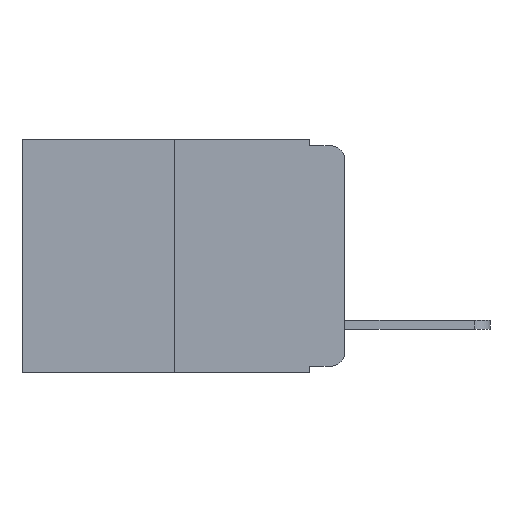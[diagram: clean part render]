
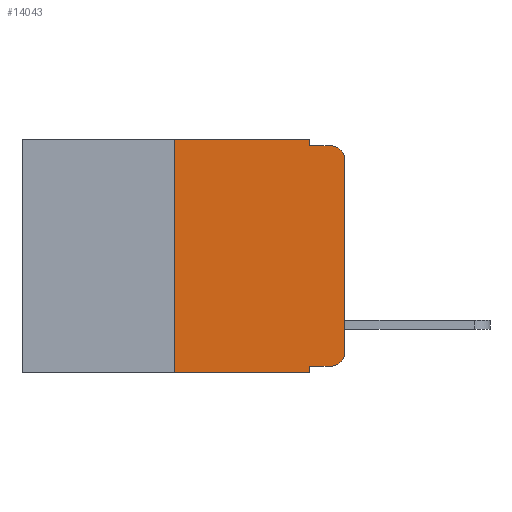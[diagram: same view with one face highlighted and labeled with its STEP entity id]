
A CAD part, left-side view. The second image highlights one B-rep face of the part: STEP entity #14043.
In plain terms, the highlighted planar face has unit normal (-1, 0, 0).
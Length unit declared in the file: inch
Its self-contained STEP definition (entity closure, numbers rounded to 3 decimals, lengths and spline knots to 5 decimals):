
#195 = EDGE_LOOP ( 'NONE', ( #18571, #7631, #4235, #989, #2558, #16724, #2683, #9960, #5244, #7052 ) ) ;
#452 = CARTESIAN_POINT ( 'NONE',  ( 0., 0.02, -0.313 ) ) ;
#512 = LINE ( 'NONE', #7724, #20447 ) ;
#828 = DIRECTION ( 'NONE',  ( 0., -1., 0. ) ) ;
#964 = PLANE ( 'NONE',  #19496 ) ;
#989 = ORIENTED_EDGE ( 'NONE', *, *, #19627, .F. ) ;
#1216 = VERTEX_POINT ( 'NONE', #5157 ) ;
#1933 = CIRCLE ( 'NONE', #14269, 0.02 ) ;
#1950 = DIRECTION ( 'NONE',  ( 0., -1., 0. ) ) ;
#2194 = CARTESIAN_POINT ( 'NONE',  ( 0., 0.25, 0. ) ) ;
#2334 = LINE ( 'NONE', #4657, #20256 ) ;
#2558 = ORIENTED_EDGE ( 'NONE', *, *, #17556, .F. ) ;
#2683 = ORIENTED_EDGE ( 'NONE', *, *, #14596, .T. ) ;
#2744 = DIRECTION ( 'NONE',  ( 0., 0., 1. ) ) ;
#3014 = CARTESIAN_POINT ( 'NONE',  ( 0., 0.051, 0. ) ) ;
#3186 = VECTOR ( 'NONE', #17641, 39.37008 ) ;
#3468 = CARTESIAN_POINT ( 'NONE',  ( 0., 0.051, 0. ) ) ;
#3731 = CARTESIAN_POINT ( 'NONE',  ( 0., 0.051, -0.01 ) ) ;
#4235 = ORIENTED_EDGE ( 'NONE', *, *, #6554, .F. ) ;
#4364 = LINE ( 'NONE', #3014, #3186 ) ;
#4483 = VERTEX_POINT ( 'NONE', #22916 ) ;
#4657 = CARTESIAN_POINT ( 'NONE',  ( 0., 0.25, 0. ) ) ;
#5157 = CARTESIAN_POINT ( 'NONE',  ( 0., 0., -0.313 ) ) ;
#5244 = ORIENTED_EDGE ( 'NONE', *, *, #22789, .T. ) ;
#5280 = EDGE_CURVE ( 'NONE', #9098, #6123, #23330, .T. ) ;
#5577 = VECTOR ( 'NONE', #2744, 39.37008 ) ;
#5737 = DIRECTION ( 'NONE',  ( 0., 0., -1. ) ) ;
#6123 = VERTEX_POINT ( 'NONE', #22788 ) ;
#6309 = CARTESIAN_POINT ( 'NONE',  ( 0., 0.051, -0.333 ) ) ;
#6348 = CARTESIAN_POINT ( 'NONE',  ( 0., 0.473, -0.343 ) ) ;
#6554 = EDGE_CURVE ( 'NONE', #20117, #6123, #14080, .T. ) ;
#6727 = LINE ( 'NONE', #19148, #5577 ) ;
#7052 = ORIENTED_EDGE ( 'NONE', *, *, #12986, .T. ) ;
#7190 = AXIS2_PLACEMENT_3D ( 'NONE', #16794, #22250, #5737 ) ;
#7631 = ORIENTED_EDGE ( 'NONE', *, *, #5280, .T. ) ;
#7724 = CARTESIAN_POINT ( 'NONE',  ( 0., 0.473, 0. ) ) ;
#7824 = DIRECTION ( 'NONE',  ( 0., 0., -1. ) ) ;
#7950 = CARTESIAN_POINT ( 'NONE',  ( 0., 0.051, -0.01 ) ) ;
#8031 = CARTESIAN_POINT ( 'NONE',  ( 0., 0.051, -0.343 ) ) ;
#8293 = DIRECTION ( 'NONE',  ( 0., -1., 0. ) ) ;
#8759 = CARTESIAN_POINT ( 'NONE',  ( 0., 0.051, 0. ) ) ;
#9098 = VERTEX_POINT ( 'NONE', #14628 ) ;
#9717 = VECTOR ( 'NONE', #828, 39.37008 ) ;
#9925 = VECTOR ( 'NONE', #14718, 39.37008 ) ;
#9960 = ORIENTED_EDGE ( 'NONE', *, *, #18666, .F. ) ;
#11906 = DIRECTION ( 'NONE',  ( 0., 0., -1. ) ) ;
#12283 = DIRECTION ( 'NONE',  ( 0., 0., 1. ) ) ;
#12408 = CARTESIAN_POINT ( 'NONE',  ( 0., 0.25, -0.343 ) ) ;
#12721 = VECTOR ( 'NONE', #8293, 39.37008 ) ;
#12986 = EDGE_CURVE ( 'NONE', #20449, #1216, #1933, .T. ) ;
#14043 = ADVANCED_FACE ( 'NONE', ( #22666 ), #964, .F. ) ;
#14080 = LINE ( 'NONE', #3731, #23258 ) ;
#14269 = AXIS2_PLACEMENT_3D ( 'NONE', #452, #15175, #7824 ) ;
#14411 = CARTESIAN_POINT ( 'NONE',  ( 0., 0.02, -0.333 ) ) ;
#14596 = EDGE_CURVE ( 'NONE', #22469, #20264, #19023, .T. ) ;
#14628 = CARTESIAN_POINT ( 'NONE',  ( 0., 0., -0.03 ) ) ;
#14718 = DIRECTION ( 'NONE',  ( 0., 0., -1. ) ) ;
#14820 = LINE ( 'NONE', #3468, #9925 ) ;
#15175 = DIRECTION ( 'NONE',  ( -1., 0., 0. ) ) ;
#16724 = ORIENTED_EDGE ( 'NONE', *, *, #19689, .F. ) ;
#16794 = CARTESIAN_POINT ( 'NONE',  ( 0., 0.02, -0.03 ) ) ;
#17201 = LINE ( 'NONE', #6309, #9717 ) ;
#17556 = EDGE_CURVE ( 'NONE', #21214, #22416, #512, .T. ) ;
#17574 = CARTESIAN_POINT ( 'NONE',  ( 0., 0.473, 0. ) ) ;
#17641 = DIRECTION ( 'NONE',  ( 0., 0., -1. ) ) ;
#18402 = EDGE_CURVE ( 'NONE', #1216, #9098, #6727, .T. ) ;
#18571 = ORIENTED_EDGE ( 'NONE', *, *, #18402, .T. ) ;
#18666 = EDGE_CURVE ( 'NONE', #4483, #20264, #14820, .T. ) ;
#19023 = LINE ( 'NONE', #6348, #12721 ) ;
#19113 = DIRECTION ( 'NONE',  ( 1., 0., 0. ) ) ;
#19148 = CARTESIAN_POINT ( 'NONE',  ( 0., 0., 0. ) ) ;
#19496 = AXIS2_PLACEMENT_3D ( 'NONE', #17574, #19113, #11906 ) ;
#19627 = EDGE_CURVE ( 'NONE', #22416, #20117, #4364, .T. ) ;
#19689 = EDGE_CURVE ( 'NONE', #22469, #21214, #2334, .T. ) ;
#20117 = VERTEX_POINT ( 'NONE', #7950 ) ;
#20256 = VECTOR ( 'NONE', #12283, 39.37008 ) ;
#20264 = VERTEX_POINT ( 'NONE', #8031 ) ;
#20447 = VECTOR ( 'NONE', #23601, 39.37008 ) ;
#20449 = VERTEX_POINT ( 'NONE', #14411 ) ;
#21214 = VERTEX_POINT ( 'NONE', #2194 ) ;
#22250 = DIRECTION ( 'NONE',  ( -1., 0., 0. ) ) ;
#22416 = VERTEX_POINT ( 'NONE', #8759 ) ;
#22469 = VERTEX_POINT ( 'NONE', #12408 ) ;
#22666 = FACE_OUTER_BOUND ( 'NONE', #195, .T. ) ;
#22788 = CARTESIAN_POINT ( 'NONE',  ( 0., 0.02, -0.01 ) ) ;
#22789 = EDGE_CURVE ( 'NONE', #4483, #20449, #17201, .T. ) ;
#22916 = CARTESIAN_POINT ( 'NONE',  ( 0., 0.051, -0.333 ) ) ;
#23258 = VECTOR ( 'NONE', #1950, 39.37008 ) ;
#23330 = CIRCLE ( 'NONE', #7190, 0.02 ) ;
#23601 = DIRECTION ( 'NONE',  ( 0., -1., 0. ) ) ;
